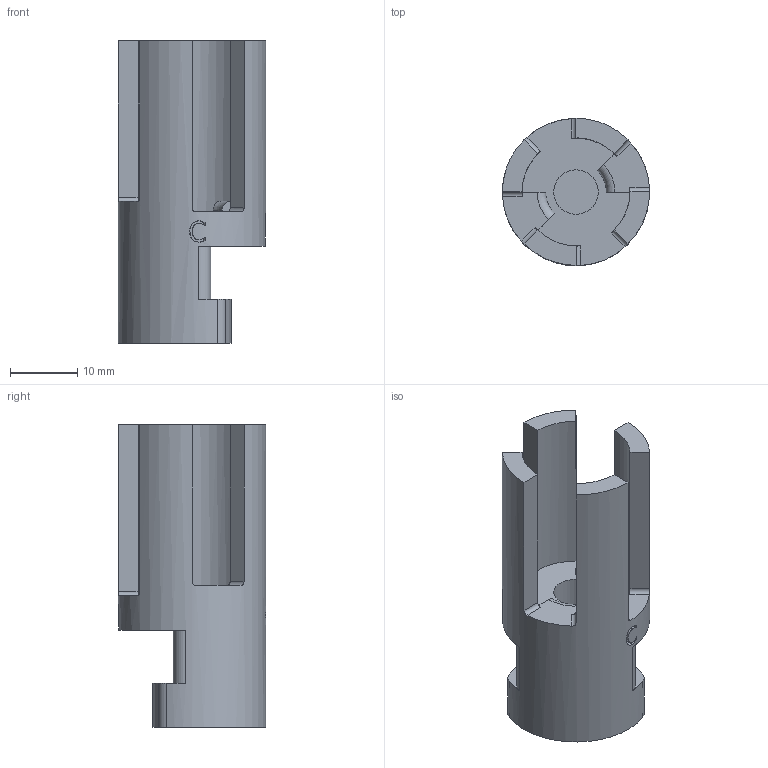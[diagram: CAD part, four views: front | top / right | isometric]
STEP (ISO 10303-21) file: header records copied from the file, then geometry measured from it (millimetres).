
FILE_DESCRIPTION(/* description */ (''),/* implementation_level */ '2;1');
FILE_NAME(/* name */ 'Chambering End Pilot Inch (0.250in).stp',/* time_stamp */ '2021-02-15T01:56:25-06:00',/* author */ ('johne'),/* organization */ (''),/* preprocessor_version */ 'ST-DEVELOPER v18',/* originating_system */ 'Autodesk Inventor 2020',/* authorisation */ '');
FILE_SCHEMA (('AUTOMOTIVE_DESIGN { 1 0 10303 214 3 1 1 }'));
Length unit declared in the file: millimetre
Products named in the file (1): chambering Tool 250 rod
Bounding box: 21.84 x 21.84 x 44.91 mm (x, y, z)
Volume: 6289.1 mm3; surface area: 4203.1 mm2
Topology: 1 solids, 1 shells, 67 faces, 192 edges, 128 vertices
Faces by surface type: plane 23, cylinder 22, bspline 20, torus 2
Full cylindrical faces by diameter (mm): 6.604 x1, 21.844 x1
Entity records: 2823 total; most frequent: CARTESIAN_POINT 1144, ORIENTED_EDGE 384, DIRECTION 280, EDGE_CURVE 192, VERTEX_POINT 128, AXIS2_PLACEMENT_3D 96, LINE 88, VECTOR 88
